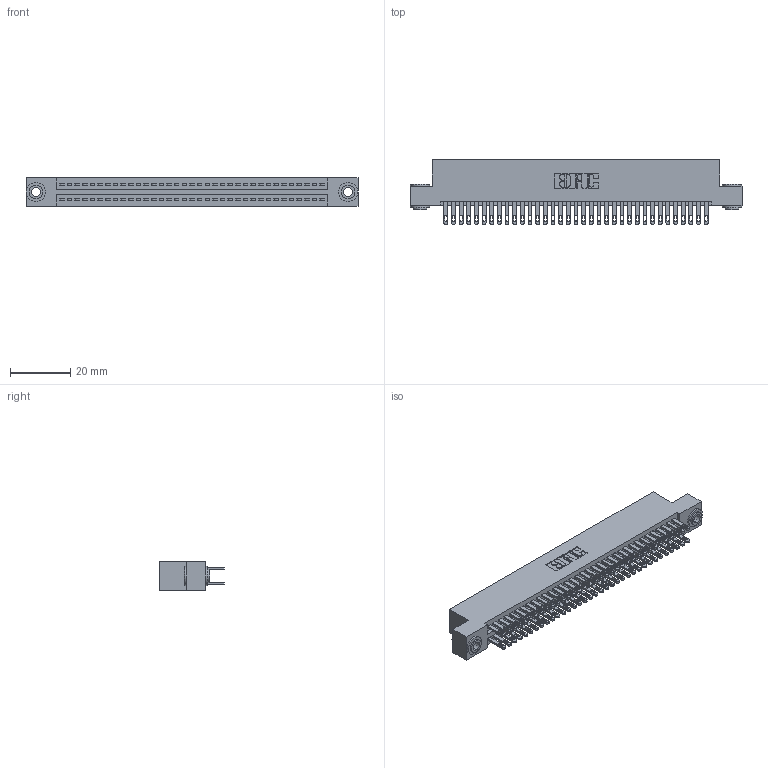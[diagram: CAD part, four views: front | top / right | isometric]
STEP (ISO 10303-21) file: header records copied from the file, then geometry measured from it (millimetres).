
FILE_DESCRIPTION (( 'STEP AP203' ), '1' );
FILE_NAME ('345-070-500-203.STEP', '2019-10-30T23:27:20', ( '' ), ( '' ), 'SwSTEP 2.0', 'SolidWorks 2016', '' );
FILE_SCHEMA (( 'CONFIG_CONTROL_DESIGN' ));
Length unit declared in the file: inch
Products named in the file (4): 345-070-500-203; 345 Part_Flush Mounting Lugs - 0.156 Dia-TH; 345-292-001_345-293-100; 345-250-002_345-250-002-102
Assembly tree (73 placements, depth 2):
  345-070-500-203
    345 Part_Flush Mounting Lugs - 0.156 Dia-TH
    345-292-001_345-293-100  x70
    345-250-002_345-250-002-102  x2
Bounding box: 110.11 x 21.51 x 9.4 mm (x, y, z)
Volume: 10864.4 mm3; surface area: 16842.7 mm2
Topology: 73 solids, 73 shells, 3384 faces, 10287 edges, 6854 vertices
Faces by surface type: plane 1980, cylinder 1396, cone 8
Entity records: 28984 total; most frequent: CARTESIAN_POINT 4839, ORIENTED_EDGE 4766, DIRECTION 4309, EDGE_CURVE 2383, VECTOR 2083, LINE 2083, VERTEX_POINT 1586, AXIS2_PLACEMENT_3D 1113
